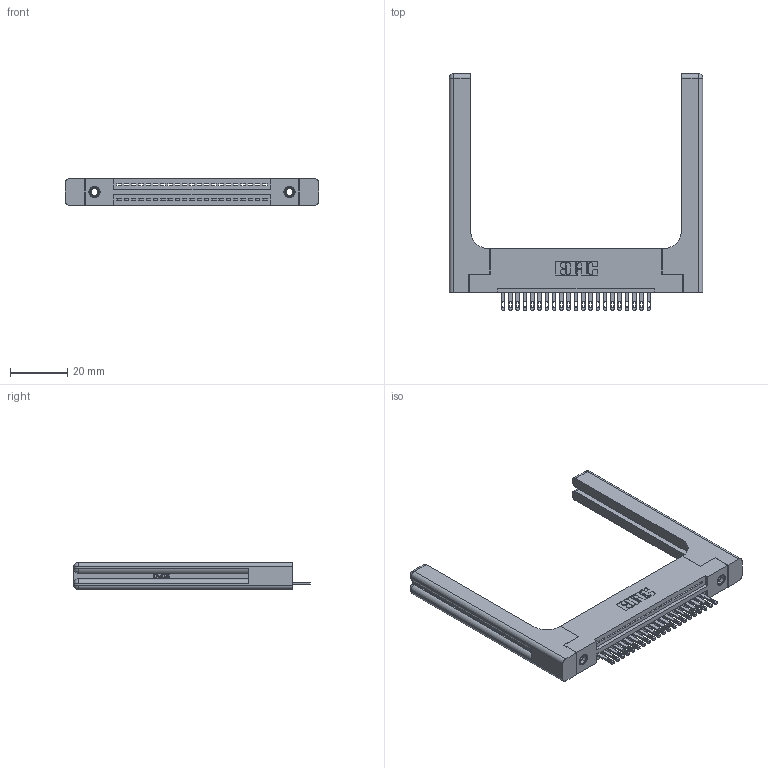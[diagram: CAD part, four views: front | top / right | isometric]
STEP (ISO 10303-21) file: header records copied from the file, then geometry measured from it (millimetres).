
FILE_DESCRIPTION (( 'STEP AP203' ), '1' );
FILE_NAME ('345-021-500-158.STEP', '2019-10-04T21:33:03', ( '' ), ( '' ), 'SwSTEP 2.0', 'SolidWorks 2016', '' );
FILE_SCHEMA (( 'CONFIG_CONTROL_DESIGN' ));
Length unit declared in the file: inch
Products named in the file (5): 345-250-001_345-250-001-102; 345-021-500-158; 345-292-001_345-293-100; 345 Part_Flush Mounting Lugs - 0.156 Dia-TH; 345-220-058_345-220-058
Assembly tree (26 placements, depth 2):
  345-021-500-158
    345 Part_Flush Mounting Lugs - 0.156 Dia-TH
    345-292-001_345-293-100  x21
    345-250-001_345-250-001-102  x2
    345-220-058_345-220-058  x2
Bounding box: 88.37 x 82.47 x 9.4 mm (x, y, z)
Volume: 16739.1 mm3; surface area: 16009.7 mm2
Topology: 26 solids, 26 shells, 1516 faces, 4535 edges, 3002 vertices
Faces by surface type: plane 942, cylinder 514, bspline 36, cone 12, sphere 8, torus 4
Entity records: 23744 total; most frequent: CARTESIAN_POINT 5084, ORIENTED_EDGE 3836, DIRECTION 3420, EDGE_CURVE 1918, LINE 1606, VECTOR 1606, VERTEX_POINT 1270, AXIS2_PLACEMENT_3D 907
